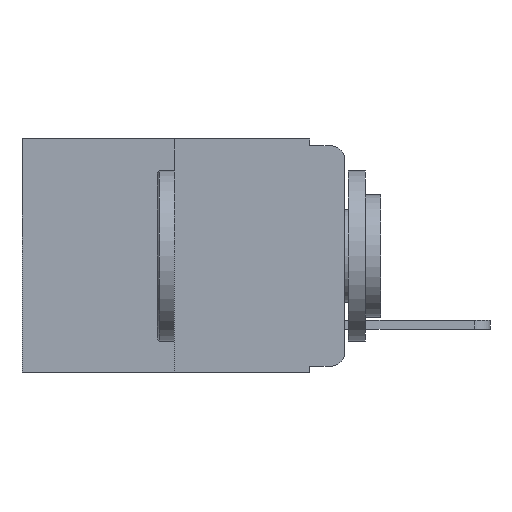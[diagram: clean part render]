
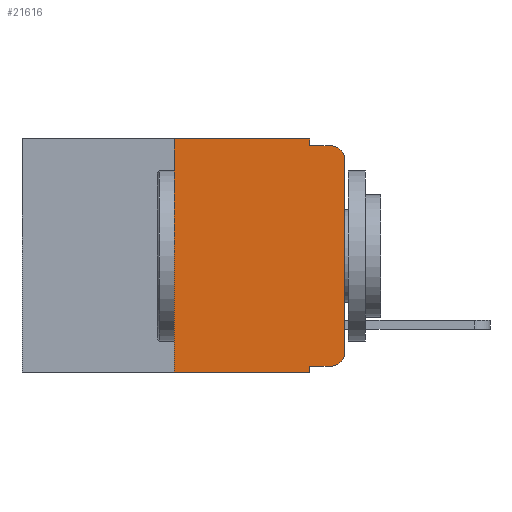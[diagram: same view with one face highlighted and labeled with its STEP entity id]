
A CAD part, left-side view. The second image highlights one B-rep face of the part: STEP entity #21616.
In plain terms, the highlighted planar face has unit normal (-1, 0, 0).
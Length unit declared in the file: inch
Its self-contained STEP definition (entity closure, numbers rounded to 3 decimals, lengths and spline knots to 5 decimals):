
#188 = DIRECTION ( 'NONE',  ( 0., 0., -1. ) ) ;
#250 = EDGE_CURVE ( 'NONE', #742, #8146, #19614, .T. ) ;
#375 = VERTEX_POINT ( 'NONE', #15714 ) ;
#395 = LINE ( 'NONE', #9889, #17120 ) ;
#742 = VERTEX_POINT ( 'NONE', #19450 ) ;
#873 = CARTESIAN_POINT ( 'NONE',  ( 0., 0.051, -0.01 ) ) ;
#1207 = ORIENTED_EDGE ( 'NONE', *, *, #11873, .F. ) ;
#1301 = DIRECTION ( 'NONE',  ( 0., -1., 0. ) ) ;
#1471 = VECTOR ( 'NONE', #13460, 39.37008 ) ;
#1535 = DIRECTION ( 'NONE',  ( 0., -1., 0. ) ) ;
#1822 = ORIENTED_EDGE ( 'NONE', *, *, #10131, .F. ) ;
#1879 = EDGE_CURVE ( 'NONE', #14660, #8053, #12610, .T. ) ;
#2463 = CARTESIAN_POINT ( 'NONE',  ( 0., 0., -0.03 ) ) ;
#2551 = LINE ( 'NONE', #7099, #19733 ) ;
#2988 = ORIENTED_EDGE ( 'NONE', *, *, #11353, .T. ) ;
#3104 = VERTEX_POINT ( 'NONE', #873 ) ;
#3578 = CARTESIAN_POINT ( 'NONE',  ( 0., 0.473, 0. ) ) ;
#3745 = CARTESIAN_POINT ( 'NONE',  ( 0., 0.051, -0.01 ) ) ;
#3960 = CARTESIAN_POINT ( 'NONE',  ( 0., 0.051, 0. ) ) ;
#3983 = VERTEX_POINT ( 'NONE', #17434 ) ;
#4752 = ORIENTED_EDGE ( 'NONE', *, *, #250, .T. ) ;
#4906 = DIRECTION ( 'NONE',  ( 0., 0., 1. ) ) ;
#5598 = ORIENTED_EDGE ( 'NONE', *, *, #7234, .T. ) ;
#5622 = DIRECTION ( 'NONE',  ( 0., -1., 0. ) ) ;
#6383 = LINE ( 'NONE', #15026, #1471 ) ;
#6887 = DIRECTION ( 'NONE',  ( 0., 0., -1. ) ) ;
#7099 = CARTESIAN_POINT ( 'NONE',  ( 0., 0.25, 0. ) ) ;
#7230 = DIRECTION ( 'NONE',  ( 1., 0., 0. ) ) ;
#7234 = EDGE_CURVE ( 'NONE', #8146, #14660, #19483, .T. ) ;
#8053 = VERTEX_POINT ( 'NONE', #20251 ) ;
#8146 = VERTEX_POINT ( 'NONE', #20364 ) ;
#8534 = CARTESIAN_POINT ( 'NONE',  ( 0., 0.473, -0.343 ) ) ;
#8849 = VECTOR ( 'NONE', #1535, 39.37008 ) ;
#8861 = ORIENTED_EDGE ( 'NONE', *, *, #18969, .T. ) ;
#9190 = EDGE_LOOP ( 'NONE', ( #5598, #14524, #18711, #1207, #1822, #11195, #2988, #20973, #8861, #4752 ) ) ;
#9373 = LINE ( 'NONE', #19895, #8849 ) ;
#9505 = VERTEX_POINT ( 'NONE', #13414 ) ;
#9812 = CARTESIAN_POINT ( 'NONE',  ( 0., 0.051, -0.333 ) ) ;
#9889 = CARTESIAN_POINT ( 'NONE',  ( 0., 0.051, 0. ) ) ;
#10131 = EDGE_CURVE ( 'NONE', #3983, #9505, #9373, .T. ) ;
#10542 = LINE ( 'NONE', #8534, #13869 ) ;
#10657 = DIRECTION ( 'NONE',  ( -1., 0., 0. ) ) ;
#10711 = AXIS2_PLACEMENT_3D ( 'NONE', #3578, #7230, #18615 ) ;
#11195 = ORIENTED_EDGE ( 'NONE', *, *, #11467, .F. ) ;
#11353 = EDGE_CURVE ( 'NONE', #15717, #375, #10542, .T. ) ;
#11467 = EDGE_CURVE ( 'NONE', #15717, #3983, #2551, .T. ) ;
#11547 = DIRECTION ( 'NONE',  ( -1., 0., 0. ) ) ;
#11873 = EDGE_CURVE ( 'NONE', #9505, #3104, #395, .T. ) ;
#12142 = DIRECTION ( 'NONE',  ( 0., 0., 1. ) ) ;
#12610 = CIRCLE ( 'NONE', #18820, 0.02 ) ;
#12622 = CARTESIAN_POINT ( 'NONE',  ( 0., 0.02, -0.03 ) ) ;
#12824 = FACE_OUTER_BOUND ( 'NONE', #9190, .T. ) ;
#13414 = CARTESIAN_POINT ( 'NONE',  ( 0., 0.051, 0. ) ) ;
#13460 = DIRECTION ( 'NONE',  ( 0., -1., 0. ) ) ;
#13869 = VECTOR ( 'NONE', #1301, 39.37008 ) ;
#13899 = VECTOR ( 'NONE', #5622, 39.37008 ) ;
#13905 = LINE ( 'NONE', #3960, #17660 ) ;
#14419 = DIRECTION ( 'NONE',  ( 0., 0., -1. ) ) ;
#14524 = ORIENTED_EDGE ( 'NONE', *, *, #1879, .T. ) ;
#14660 = VERTEX_POINT ( 'NONE', #2463 ) ;
#15026 = CARTESIAN_POINT ( 'NONE',  ( 0., 0.051, -0.333 ) ) ;
#15089 = CARTESIAN_POINT ( 'NONE',  ( 0., 0.02, -0.313 ) ) ;
#15354 = VECTOR ( 'NONE', #4906, 39.37008 ) ;
#15714 = CARTESIAN_POINT ( 'NONE',  ( 0., 0.051, -0.343 ) ) ;
#15717 = VERTEX_POINT ( 'NONE', #18170 ) ;
#16500 = VERTEX_POINT ( 'NONE', #9812 ) ;
#16587 = CARTESIAN_POINT ( 'NONE',  ( 0., 0., 0. ) ) ;
#16912 = EDGE_CURVE ( 'NONE', #16500, #375, #13905, .T. ) ;
#17120 = VECTOR ( 'NONE', #20963, 39.37008 ) ;
#17434 = CARTESIAN_POINT ( 'NONE',  ( 0., 0.25, 0. ) ) ;
#17660 = VECTOR ( 'NONE', #188, 39.37008 ) ;
#18041 = AXIS2_PLACEMENT_3D ( 'NONE', #15089, #10657, #6887 ) ;
#18140 = LINE ( 'NONE', #3745, #13899 ) ;
#18170 = CARTESIAN_POINT ( 'NONE',  ( 0., 0.25, -0.343 ) ) ;
#18615 = DIRECTION ( 'NONE',  ( 0., 0., -1. ) ) ;
#18711 = ORIENTED_EDGE ( 'NONE', *, *, #20665, .F. ) ;
#18820 = AXIS2_PLACEMENT_3D ( 'NONE', #12622, #11547, #14419 ) ;
#18969 = EDGE_CURVE ( 'NONE', #16500, #742, #6383, .T. ) ;
#19450 = CARTESIAN_POINT ( 'NONE',  ( 0., 0.02, -0.333 ) ) ;
#19483 = LINE ( 'NONE', #16587, #15354 ) ;
#19614 = CIRCLE ( 'NONE', #18041, 0.02 ) ;
#19733 = VECTOR ( 'NONE', #12142, 39.37008 ) ;
#19895 = CARTESIAN_POINT ( 'NONE',  ( 0., 0.473, 0. ) ) ;
#20025 = PLANE ( 'NONE',  #10711 ) ;
#20251 = CARTESIAN_POINT ( 'NONE',  ( 0., 0.02, -0.01 ) ) ;
#20364 = CARTESIAN_POINT ( 'NONE',  ( 0., 0., -0.313 ) ) ;
#20665 = EDGE_CURVE ( 'NONE', #3104, #8053, #18140, .T. ) ;
#20963 = DIRECTION ( 'NONE',  ( 0., 0., -1. ) ) ;
#20973 = ORIENTED_EDGE ( 'NONE', *, *, #16912, .F. ) ;
#21616 = ADVANCED_FACE ( 'NONE', ( #12824 ), #20025, .F. ) ;
